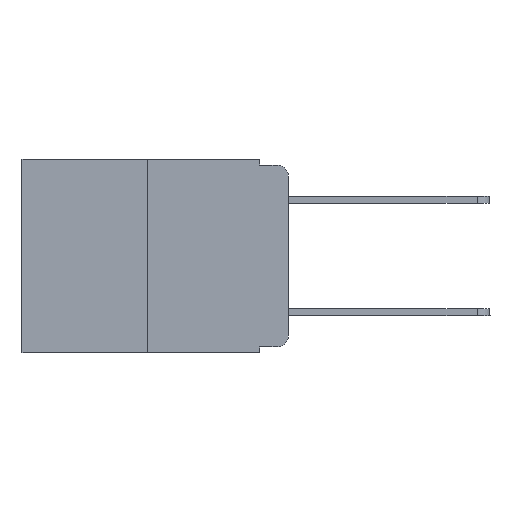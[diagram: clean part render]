
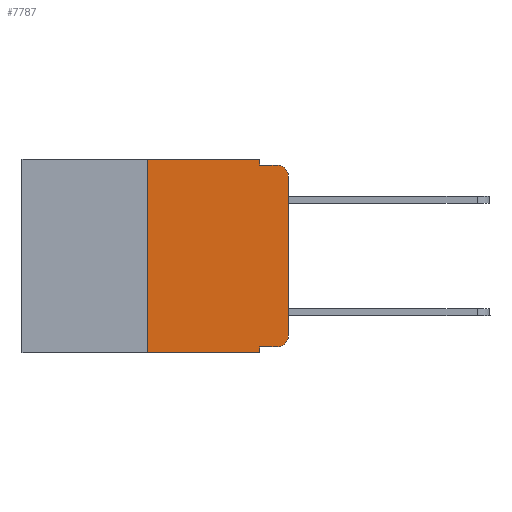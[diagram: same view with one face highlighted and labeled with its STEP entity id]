
A CAD part, left-side view. The second image highlights one B-rep face of the part: STEP entity #7787.
In plain terms, the highlighted planar face has unit normal (-1, 0, 0).
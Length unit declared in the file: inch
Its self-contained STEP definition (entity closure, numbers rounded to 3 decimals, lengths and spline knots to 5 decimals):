
#11 = EDGE_CURVE ( 'NONE', #11328, #18641, #16033, .T. ) ;
#153 = EDGE_CURVE ( 'NONE', #23780, #23741, #11287, .T. ) ;
#505 = CARTESIAN_POINT ( 'NONE',  ( 0., 0.473, 0. ) ) ;
#520 = VECTOR ( 'NONE', #9807, 39.37008 ) ;
#693 = LINE ( 'NONE', #944, #8812 ) ;
#944 = CARTESIAN_POINT ( 'NONE',  ( 0., 0.051, 0. ) ) ;
#1202 = FACE_OUTER_BOUND ( 'NONE', #8126, .T. ) ;
#1689 = VECTOR ( 'NONE', #23474, 39.37008 ) ;
#2130 = EDGE_CURVE ( 'NONE', #3520, #11328, #19245, .T. ) ;
#2326 = AXIS2_PLACEMENT_3D ( 'NONE', #14059, #21091, #23029 ) ;
#2406 = CARTESIAN_POINT ( 'NONE',  ( 0., 0.051, -0.333 ) ) ;
#2518 = EDGE_CURVE ( 'NONE', #9722, #18641, #7083, .T. ) ;
#2590 = CARTESIAN_POINT ( 'NONE',  ( 0., 0.051, -0.01 ) ) ;
#2592 = ORIENTED_EDGE ( 'NONE', *, *, #11, .F. ) ;
#2606 = DIRECTION ( 'NONE',  ( 0., 0., -1. ) ) ;
#2655 = EDGE_CURVE ( 'NONE', #13732, #9722, #8168, .T. ) ;
#2848 = VECTOR ( 'NONE', #7632, 39.37008 ) ;
#2932 = DIRECTION ( 'NONE',  ( 0., -1., 0. ) ) ;
#3275 = EDGE_CURVE ( 'NONE', #21936, #3520, #4465, .T. ) ;
#3512 = ORIENTED_EDGE ( 'NONE', *, *, #23328, .F. ) ;
#3520 = VERTEX_POINT ( 'NONE', #23538 ) ;
#3788 = EDGE_CURVE ( 'NONE', #19636, #23730, #17069, .T. ) ;
#4465 = LINE ( 'NONE', #505, #4686 ) ;
#4643 = CARTESIAN_POINT ( 'NONE',  ( 0., 0., 0. ) ) ;
#4686 = VECTOR ( 'NONE', #8093, 39.37008 ) ;
#5162 = CIRCLE ( 'NONE', #8253, 0.02 ) ;
#5323 = VECTOR ( 'NONE', #21202, 39.37008 ) ;
#6263 = PLANE ( 'NONE',  #2326 ) ;
#7083 = CIRCLE ( 'NONE', #20659, 0.02 ) ;
#7473 = VECTOR ( 'NONE', #2932, 39.37008 ) ;
#7632 = DIRECTION ( 'NONE',  ( 0., -1., 0. ) ) ;
#7787 = ADVANCED_FACE ( 'NONE', ( #1202 ), #6263, .F. ) ;
#8093 = DIRECTION ( 'NONE',  ( 0., -1., 0. ) ) ;
#8126 = EDGE_LOOP ( 'NONE', ( #23187, #13359, #2592, #9969, #9607, #17255, #8203, #3512, #13787, #17644 ) ) ;
#8168 = LINE ( 'NONE', #4643, #1689 ) ;
#8203 = ORIENTED_EDGE ( 'NONE', *, *, #153, .T. ) ;
#8253 = AXIS2_PLACEMENT_3D ( 'NONE', #18427, #16484, #14559 ) ;
#8271 = CARTESIAN_POINT ( 'NONE',  ( 0., 0.02, -0.01 ) ) ;
#8812 = VECTOR ( 'NONE', #20713, 39.37008 ) ;
#9053 = CARTESIAN_POINT ( 'NONE',  ( 0., 0., -0.313 ) ) ;
#9144 = CARTESIAN_POINT ( 'NONE',  ( 0., 0., -0.03 ) ) ;
#9291 = CARTESIAN_POINT ( 'NONE',  ( 0., 0.25, 0. ) ) ;
#9415 = CARTESIAN_POINT ( 'NONE',  ( 0., 0.25, 0. ) ) ;
#9607 = ORIENTED_EDGE ( 'NONE', *, *, #3275, .F. ) ;
#9722 = VERTEX_POINT ( 'NONE', #9144 ) ;
#9807 = DIRECTION ( 'NONE',  ( 0., -1., 0. ) ) ;
#9969 = ORIENTED_EDGE ( 'NONE', *, *, #2130, .F. ) ;
#11118 = DIRECTION ( 'NONE',  ( 0., 0., 1. ) ) ;
#11287 = LINE ( 'NONE', #16497, #2848 ) ;
#11328 = VERTEX_POINT ( 'NONE', #2590 ) ;
#13064 = LINE ( 'NONE', #9415, #22141 ) ;
#13359 = ORIENTED_EDGE ( 'NONE', *, *, #2518, .T. ) ;
#13652 = DIRECTION ( 'NONE',  ( -1., 0., 0. ) ) ;
#13732 = VERTEX_POINT ( 'NONE', #9053 ) ;
#13787 = ORIENTED_EDGE ( 'NONE', *, *, #3788, .T. ) ;
#14059 = CARTESIAN_POINT ( 'NONE',  ( 0., 0.473, 0. ) ) ;
#14559 = DIRECTION ( 'NONE',  ( 0., 0., -1. ) ) ;
#15052 = EDGE_CURVE ( 'NONE', #23780, #21936, #13064, .T. ) ;
#15087 = CARTESIAN_POINT ( 'NONE',  ( 0., 0.051, -0.343 ) ) ;
#15451 = CARTESIAN_POINT ( 'NONE',  ( 0., 0.02, -0.333 ) ) ;
#15459 = CARTESIAN_POINT ( 'NONE',  ( 0., 0.02, -0.03 ) ) ;
#16033 = LINE ( 'NONE', #19919, #7473 ) ;
#16484 = DIRECTION ( 'NONE',  ( -1., 0., 0. ) ) ;
#16497 = CARTESIAN_POINT ( 'NONE',  ( 0., 0.473, -0.343 ) ) ;
#17069 = LINE ( 'NONE', #2406, #520 ) ;
#17188 = CARTESIAN_POINT ( 'NONE',  ( 0., 0.051, 0. ) ) ;
#17255 = ORIENTED_EDGE ( 'NONE', *, *, #15052, .F. ) ;
#17644 = ORIENTED_EDGE ( 'NONE', *, *, #19340, .T. ) ;
#18427 = CARTESIAN_POINT ( 'NONE',  ( 0., 0.02, -0.313 ) ) ;
#18641 = VERTEX_POINT ( 'NONE', #8271 ) ;
#19245 = LINE ( 'NONE', #17188, #5323 ) ;
#19340 = EDGE_CURVE ( 'NONE', #23730, #13732, #5162, .T. ) ;
#19636 = VERTEX_POINT ( 'NONE', #21214 ) ;
#19919 = CARTESIAN_POINT ( 'NONE',  ( 0., 0.051, -0.01 ) ) ;
#20659 = AXIS2_PLACEMENT_3D ( 'NONE', #15459, #13652, #2606 ) ;
#20713 = DIRECTION ( 'NONE',  ( 0., 0., -1. ) ) ;
#21091 = DIRECTION ( 'NONE',  ( 1., 0., 0. ) ) ;
#21202 = DIRECTION ( 'NONE',  ( 0., 0., -1. ) ) ;
#21214 = CARTESIAN_POINT ( 'NONE',  ( 0., 0.051, -0.333 ) ) ;
#21936 = VERTEX_POINT ( 'NONE', #9291 ) ;
#22141 = VECTOR ( 'NONE', #11118, 39.37008 ) ;
#22980 = CARTESIAN_POINT ( 'NONE',  ( 0., 0.25, -0.343 ) ) ;
#23029 = DIRECTION ( 'NONE',  ( 0., 0., -1. ) ) ;
#23187 = ORIENTED_EDGE ( 'NONE', *, *, #2655, .T. ) ;
#23328 = EDGE_CURVE ( 'NONE', #19636, #23741, #693, .T. ) ;
#23474 = DIRECTION ( 'NONE',  ( 0., 0., 1. ) ) ;
#23538 = CARTESIAN_POINT ( 'NONE',  ( 0., 0.051, 0. ) ) ;
#23730 = VERTEX_POINT ( 'NONE', #15451 ) ;
#23741 = VERTEX_POINT ( 'NONE', #15087 ) ;
#23780 = VERTEX_POINT ( 'NONE', #22980 ) ;
